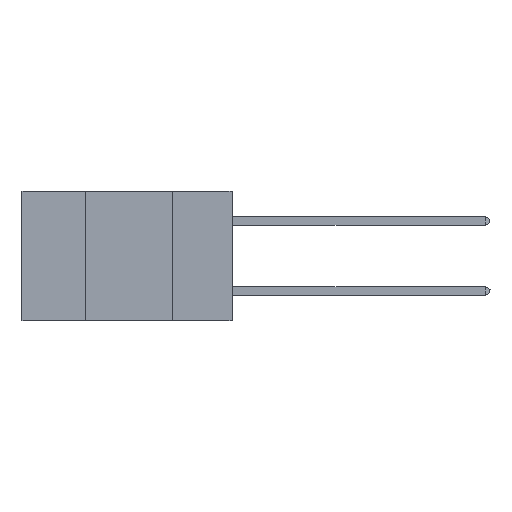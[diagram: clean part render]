
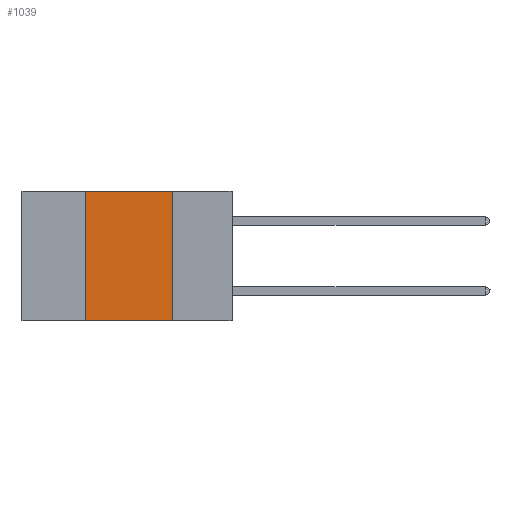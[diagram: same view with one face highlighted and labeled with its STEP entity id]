
A CAD part, left-side view. The second image highlights one B-rep face of the part: STEP entity #1039.
In plain terms, the highlighted planar face has unit normal (-1, 0, 0).
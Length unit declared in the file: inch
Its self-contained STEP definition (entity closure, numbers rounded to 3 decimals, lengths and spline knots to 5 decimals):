
#45 = DIRECTION ( 'NONE',  ( 0., 0., -1. ) ) ;
#1039 = ADVANCED_FACE ( 'NONE', ( #14415 ), #8995, .F. ) ;
#2208 = LINE ( 'NONE', #39615, #24807 ) ;
#4508 = VECTOR ( 'NONE', #15212, 39.37008 ) ;
#5030 = DIRECTION ( 'NONE',  ( 0., -1., 0. ) ) ;
#6718 = AXIS2_PLACEMENT_3D ( 'NONE', #12274, #25030, #45 ) ;
#8036 = VERTEX_POINT ( 'NONE', #38731 ) ;
#8238 = VECTOR ( 'NONE', #28006, 39.37008 ) ;
#8897 = ORIENTED_EDGE ( 'NONE', *, *, #10592, .T. ) ;
#8995 = PLANE ( 'NONE',  #6718 ) ;
#10592 = EDGE_CURVE ( 'NONE', #26583, #12547, #40075, .T. ) ;
#10910 = LINE ( 'NONE', #34125, #4508 ) ;
#12031 = VECTOR ( 'NONE', #5030, 39.37008 ) ;
#12125 = EDGE_LOOP ( 'NONE', ( #18367, #32672, #40178, #8897 ) ) ;
#12274 = CARTESIAN_POINT ( 'NONE',  ( 0., 0.6, 0. ) ) ;
#12547 = VERTEX_POINT ( 'NONE', #33106 ) ;
#13484 = EDGE_CURVE ( 'NONE', #26583, #8036, #33363, .T. ) ;
#14032 = VERTEX_POINT ( 'NONE', #37454 ) ;
#14415 = FACE_OUTER_BOUND ( 'NONE', #12125, .T. ) ;
#15212 = DIRECTION ( 'NONE',  ( 0., 0., -1. ) ) ;
#18367 = ORIENTED_EDGE ( 'NONE', *, *, #31956, .F. ) ;
#23215 = EDGE_CURVE ( 'NONE', #8036, #14032, #2208, .T. ) ;
#24807 = VECTOR ( 'NONE', #27224, 39.37008 ) ;
#25030 = DIRECTION ( 'NONE',  ( 1., 0., 0. ) ) ;
#26583 = VERTEX_POINT ( 'NONE', #33072 ) ;
#27224 = DIRECTION ( 'NONE',  ( 0., -1., 0. ) ) ;
#28006 = DIRECTION ( 'NONE',  ( 0., 0., 1. ) ) ;
#31956 = EDGE_CURVE ( 'NONE', #14032, #12547, #10910, .T. ) ;
#32672 = ORIENTED_EDGE ( 'NONE', *, *, #23215, .F. ) ;
#33072 = CARTESIAN_POINT ( 'NONE',  ( 0., 0.42, -0.37 ) ) ;
#33106 = CARTESIAN_POINT ( 'NONE',  ( 0., 0.17, -0.37 ) ) ;
#33363 = LINE ( 'NONE', #34260, #8238 ) ;
#34125 = CARTESIAN_POINT ( 'NONE',  ( 0., 0.17, 0. ) ) ;
#34260 = CARTESIAN_POINT ( 'NONE',  ( 0., 0.42, 0. ) ) ;
#37373 = CARTESIAN_POINT ( 'NONE',  ( 0., 0.6, -0.37 ) ) ;
#37454 = CARTESIAN_POINT ( 'NONE',  ( 0., 0.17, 0. ) ) ;
#38731 = CARTESIAN_POINT ( 'NONE',  ( 0., 0.42, 0. ) ) ;
#39615 = CARTESIAN_POINT ( 'NONE',  ( 0., 0.6, 0. ) ) ;
#40075 = LINE ( 'NONE', #37373, #12031 ) ;
#40178 = ORIENTED_EDGE ( 'NONE', *, *, #13484, .F. ) ;
